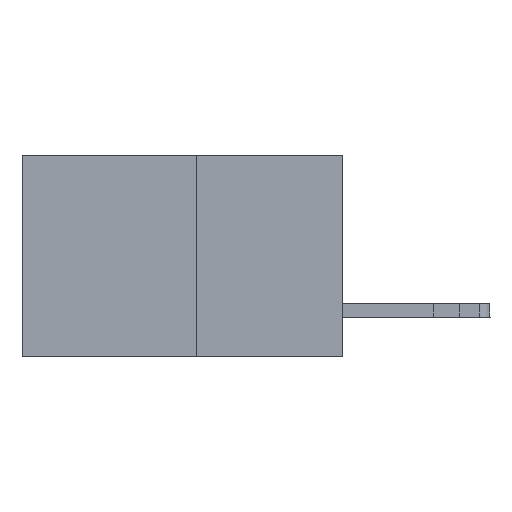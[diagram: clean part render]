
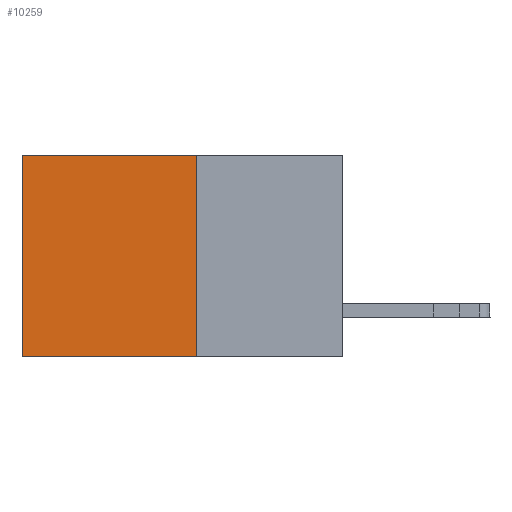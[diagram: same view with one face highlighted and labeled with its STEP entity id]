
A CAD part, left-side view. The second image highlights one B-rep face of the part: STEP entity #10259.
In plain terms, the highlighted planar face has unit normal (-1, 0, 0).
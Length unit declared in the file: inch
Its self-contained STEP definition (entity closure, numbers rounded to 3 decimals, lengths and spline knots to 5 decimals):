
#410 = DIRECTION ( 'NONE',  ( 0., 1., 0. ) ) ;
#770 = DIRECTION ( 'NONE',  ( 1., 0., 0. ) ) ;
#1757 = LINE ( 'NONE', #11457, #6564 ) ;
#2494 = AXIS2_PLACEMENT_3D ( 'NONE', #11544, #770, #13324 ) ;
#2520 = DIRECTION ( 'NONE',  ( 0., 0., -1. ) ) ;
#4346 = DIRECTION ( 'NONE',  ( 0., 0., -1. ) ) ;
#4836 = LINE ( 'NONE', #21929, #9047 ) ;
#5288 = EDGE_CURVE ( 'NONE', #14379, #11005, #14946, .T. ) ;
#6038 = VECTOR ( 'NONE', #7364, 39.37008 ) ;
#6143 = EDGE_CURVE ( 'NONE', #11005, #21133, #1757, .T. ) ;
#6564 = VECTOR ( 'NONE', #4346, 39.37008 ) ;
#6880 = VERTEX_POINT ( 'NONE', #18622 ) ;
#7364 = DIRECTION ( 'NONE',  ( 0., 1., 0. ) ) ;
#7491 = CARTESIAN_POINT ( 'NONE',  ( 0.277, 0.27, 0. ) ) ;
#8320 = ORIENTED_EDGE ( 'NONE', *, *, #5288, .T. ) ;
#9047 = VECTOR ( 'NONE', #410, 39.37008 ) ;
#9355 = ORIENTED_EDGE ( 'NONE', *, *, #13194, .F. ) ;
#10259 = ADVANCED_FACE ( 'NONE', ( #20241 ), #20441, .F. ) ;
#11005 = VERTEX_POINT ( 'NONE', #20492 ) ;
#11457 = CARTESIAN_POINT ( 'NONE',  ( 0.277, 0.59, -0.37 ) ) ;
#11544 = CARTESIAN_POINT ( 'NONE',  ( 0.277, 0.27, -0.37 ) ) ;
#11806 = ORIENTED_EDGE ( 'NONE', *, *, #21713, .F. ) ;
#11901 = CARTESIAN_POINT ( 'NONE',  ( 0.277, 0.59, -0.37 ) ) ;
#13035 = VECTOR ( 'NONE', #2520, 39.37008 ) ;
#13194 = EDGE_CURVE ( 'NONE', #6880, #21133, #4836, .T. ) ;
#13236 = EDGE_LOOP ( 'NONE', ( #15923, #9355, #11806, #8320 ) ) ;
#13289 = CARTESIAN_POINT ( 'NONE',  ( 0.277, 0.27, -0.37 ) ) ;
#13324 = DIRECTION ( 'NONE',  ( 0., 0., -1. ) ) ;
#14379 = VERTEX_POINT ( 'NONE', #7491 ) ;
#14946 = LINE ( 'NONE', #16212, #6038 ) ;
#15923 = ORIENTED_EDGE ( 'NONE', *, *, #6143, .T. ) ;
#16212 = CARTESIAN_POINT ( 'NONE',  ( 0.277, 0.27, 0. ) ) ;
#18622 = CARTESIAN_POINT ( 'NONE',  ( 0.277, 0.27, -0.37 ) ) ;
#20241 = FACE_OUTER_BOUND ( 'NONE', #13236, .T. ) ;
#20441 = PLANE ( 'NONE',  #2494 ) ;
#20492 = CARTESIAN_POINT ( 'NONE',  ( 0.277, 0.59, 0. ) ) ;
#21133 = VERTEX_POINT ( 'NONE', #11901 ) ;
#21713 = EDGE_CURVE ( 'NONE', #14379, #6880, #22609, .T. ) ;
#21929 = CARTESIAN_POINT ( 'NONE',  ( 0.277, 0.27, -0.37 ) ) ;
#22609 = LINE ( 'NONE', #13289, #13035 ) ;
